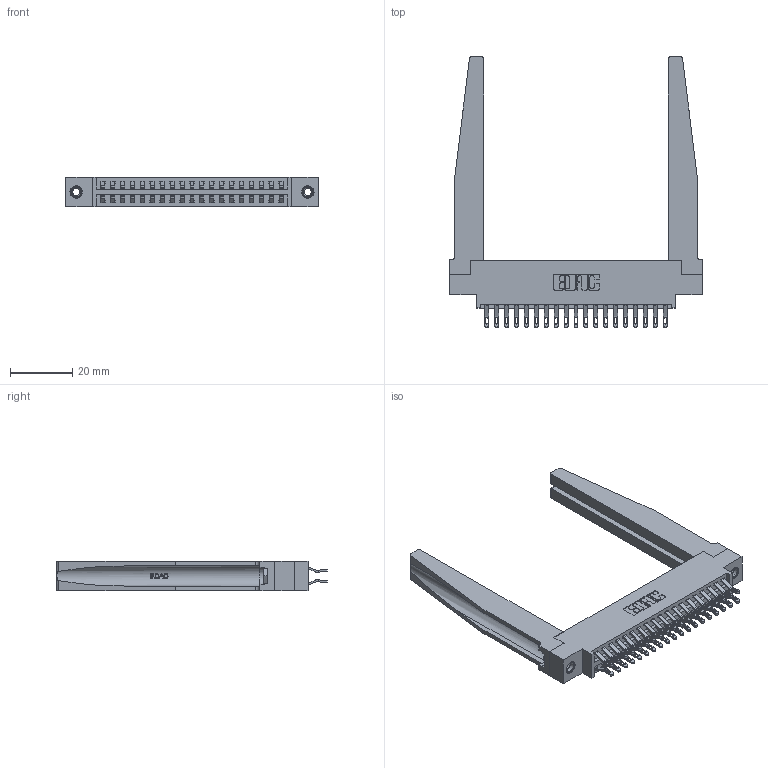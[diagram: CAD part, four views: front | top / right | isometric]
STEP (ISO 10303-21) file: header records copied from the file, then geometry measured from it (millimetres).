
FILE_DESCRIPTION (( 'STEP AP203' ), '1' );
FILE_NAME ('346-038-555-878.STEP', '2022-05-20T00:11:49', ( '' ), ( '' ), 'SwSTEP 2.0', 'SolidWorks 2020', '' );
FILE_SCHEMA (( 'CONFIG_CONTROL_DESIGN' ));
Length unit declared in the file: inch
Products named in the file (5): 346-038-555-878; 346-220-078_345-220-078; 346 Part_0.170 Offset - 0.156 Dia-TH; 345-250-001_345-250-001-102; 345-292-001_555 Tail
Assembly tree (43 placements, depth 2):
  346-038-555-878
    346 Part_0.170 Offset - 0.156 Dia-TH
    345-292-001_555 Tail  x38
    346-220-078_345-220-078  x2
    345-250-001_345-250-001-102  x2
Bounding box: 80.9 x 86.74 x 9.4 mm (x, y, z)
Volume: 14556.4 mm3; surface area: 17295.1 mm2
Topology: 43 solids, 43 shells, 2578 faces, 7939 edges, 5282 vertices
Faces by surface type: plane 1490, cylinder 1036, bspline 36, cone 12, torus 4
Entity records: 21118 total; most frequent: CARTESIAN_POINT 4491, ORIENTED_EDGE 3282, DIRECTION 2963, EDGE_CURVE 1641, VECTOR 1319, LINE 1319, VERTEX_POINT 1088, AXIS2_PLACEMENT_3D 822
